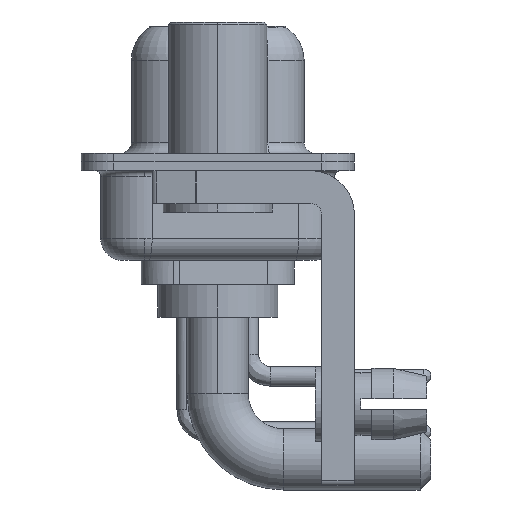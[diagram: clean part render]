
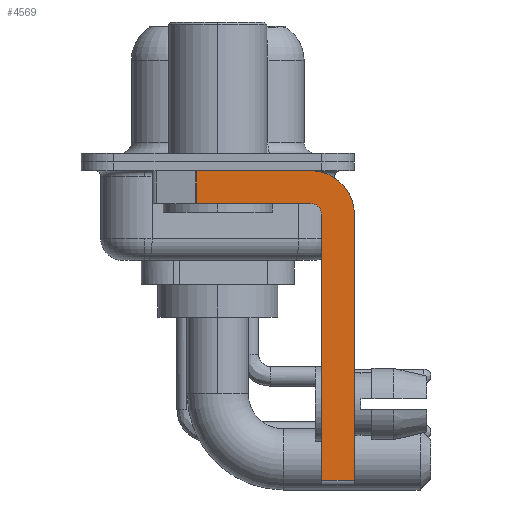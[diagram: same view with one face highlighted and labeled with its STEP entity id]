
A CAD part, left-side view. The second image highlights one B-rep face of the part: STEP entity #4569.
In plain terms, the highlighted planar face has unit normal (-1, 0, 0).
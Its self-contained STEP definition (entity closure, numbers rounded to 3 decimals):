
#668 = DIRECTION ( 'NONE',  ( 0., 0., -1. ) ) ;
#1180 = VERTEX_POINT ( 'NONE', #19474 ) ;
#1186 = DIRECTION ( 'NONE',  ( -1., 0., 0. ) ) ;
#1205 = LINE ( 'NONE', #11473, #3272 ) ;
#1273 = EDGE_CURVE ( 'NONE', #15470, #19643, #20476, .T. ) ;
#1281 = CIRCLE ( 'NONE', #15191, 0.5 ) ;
#1756 = EDGE_CURVE ( 'NONE', #1180, #3788, #4873, .T. ) ;
#1793 = AXIS2_PLACEMENT_3D ( 'NONE', #11819, #11915, #668 ) ;
#1850 = ORIENTED_EDGE ( 'NONE', *, *, #9100, .T. ) ;
#1886 = FACE_OUTER_BOUND ( 'NONE', #3737, .T. ) ;
#2085 = CARTESIAN_POINT ( 'NONE',  ( -2.9, -6.25, -2.4 ) ) ;
#2198 = DIRECTION ( 'NONE',  ( 1., 0., 0. ) ) ;
#2397 = VERTEX_POINT ( 'NONE', #4970 ) ;
#2559 = VECTOR ( 'NONE', #9668, 1000. ) ;
#2826 = VECTOR ( 'NONE', #18596, 1000. ) ;
#3000 = ORIENTED_EDGE ( 'NONE', *, *, #14231, .F. ) ;
#3191 = CARTESIAN_POINT ( 'NONE',  ( -2.9, -6.25, -2.4 ) ) ;
#3272 = VECTOR ( 'NONE', #19058, 1000. ) ;
#3725 = CARTESIAN_POINT ( 'NONE',  ( -2.9, -4.25, -14.55 ) ) ;
#3737 = EDGE_LOOP ( 'NONE', ( #13755, #11498, #6599, #9233, #5013, #1850, #3000, #14218 ) ) ;
#3788 = VERTEX_POINT ( 'NONE', #6149 ) ;
#3828 = LINE ( 'NONE', #3725, #9760 ) ;
#3864 = DIRECTION ( 'NONE',  ( 0., -1., 0. ) ) ;
#3899 = DIRECTION ( 'NONE',  ( 0., 0., -1. ) ) ;
#4243 = LINE ( 'NONE', #7425, #18964 ) ;
#4569 = ADVANCED_FACE ( 'NONE', ( #1886 ), #14953, .F. ) ;
#4873 = LINE ( 'NONE', #18169, #2826 ) ;
#4970 = CARTESIAN_POINT ( 'NONE',  ( -2.9, -4.75, -2.4 ) ) ;
#5013 = ORIENTED_EDGE ( 'NONE', *, *, #19463, .F. ) ;
#5307 = CARTESIAN_POINT ( 'NONE',  ( -2.9, -4.75, -14.55 ) ) ;
#5373 = CARTESIAN_POINT ( 'NONE',  ( -2.9, -4.25, -2.4 ) ) ;
#5404 = VERTEX_POINT ( 'NONE', #5496 ) ;
#5496 = CARTESIAN_POINT ( 'NONE',  ( -2.9, -6.25, -14.55 ) ) ;
#6149 = CARTESIAN_POINT ( 'NONE',  ( -2.9, 0.978, -1.9 ) ) ;
#6599 = ORIENTED_EDGE ( 'NONE', *, *, #15989, .F. ) ;
#6945 = LINE ( 'NONE', #10340, #20502 ) ;
#7425 = CARTESIAN_POINT ( 'NONE',  ( -2.9, -4.75, -14.8 ) ) ;
#8752 = EDGE_CURVE ( 'NONE', #2397, #21011, #1281, .T. ) ;
#9016 = DIRECTION ( 'NONE',  ( 0., -1., 0. ) ) ;
#9100 = EDGE_CURVE ( 'NONE', #20748, #5404, #3828, .T. ) ;
#9233 = ORIENTED_EDGE ( 'NONE', *, *, #8752, .F. ) ;
#9668 = DIRECTION ( 'NONE',  ( 0., 0., -1. ) ) ;
#9760 = VECTOR ( 'NONE', #9016, 1000. ) ;
#9854 = CARTESIAN_POINT ( 'NONE',  ( -2.9, -4.25, -1.9 ) ) ;
#10340 = CARTESIAN_POINT ( 'NONE',  ( -2.9, 3., -0.4 ) ) ;
#10717 = DIRECTION ( 'NONE',  ( 0., 0., 1. ) ) ;
#11337 = AXIS2_PLACEMENT_3D ( 'NONE', #5373, #2198, #3899 ) ;
#11473 = CARTESIAN_POINT ( 'NONE',  ( -2.9, -4.25, -1.9 ) ) ;
#11498 = ORIENTED_EDGE ( 'NONE', *, *, #1756, .T. ) ;
#11819 = CARTESIAN_POINT ( 'NONE',  ( -2.9, -4.25, -2.4 ) ) ;
#11915 = DIRECTION ( 'NONE',  ( 1., 0., 0. ) ) ;
#12344 = EDGE_CURVE ( 'NONE', #1180, #15470, #6945, .T. ) ;
#13632 = CARTESIAN_POINT ( 'NONE',  ( -2.9, -4.25, -0.4 ) ) ;
#13755 = ORIENTED_EDGE ( 'NONE', *, *, #12344, .F. ) ;
#14159 = CARTESIAN_POINT ( 'NONE',  ( -2.9, -4.25, -2.4 ) ) ;
#14218 = ORIENTED_EDGE ( 'NONE', *, *, #1273, .F. ) ;
#14231 = EDGE_CURVE ( 'NONE', #19643, #5404, #19349, .T. ) ;
#14953 = PLANE ( 'NONE',  #11337 ) ;
#15191 = AXIS2_PLACEMENT_3D ( 'NONE', #14159, #1186, #15629 ) ;
#15470 = VERTEX_POINT ( 'NONE', #13632 ) ;
#15629 = DIRECTION ( 'NONE',  ( 0., 0., 1. ) ) ;
#15989 = EDGE_CURVE ( 'NONE', #21011, #3788, #1205, .T. ) ;
#18169 = CARTESIAN_POINT ( 'NONE',  ( -2.9, 0.978, -1.9 ) ) ;
#18596 = DIRECTION ( 'NONE',  ( 0., 0., -1. ) ) ;
#18964 = VECTOR ( 'NONE', #10717, 1000. ) ;
#19058 = DIRECTION ( 'NONE',  ( 0., 1., 0. ) ) ;
#19349 = LINE ( 'NONE', #3191, #2559 ) ;
#19463 = EDGE_CURVE ( 'NONE', #20748, #2397, #4243, .T. ) ;
#19474 = CARTESIAN_POINT ( 'NONE',  ( -2.9, 0.978, -0.4 ) ) ;
#19643 = VERTEX_POINT ( 'NONE', #2085 ) ;
#20476 = CIRCLE ( 'NONE', #1793, 2. ) ;
#20502 = VECTOR ( 'NONE', #3864, 1000. ) ;
#20748 = VERTEX_POINT ( 'NONE', #5307 ) ;
#21011 = VERTEX_POINT ( 'NONE', #9854 ) ;
